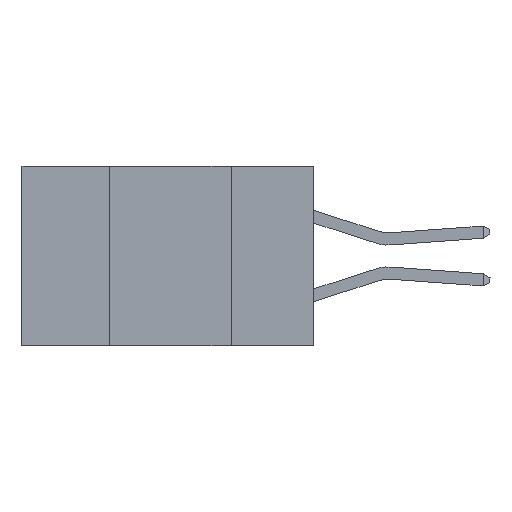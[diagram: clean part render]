
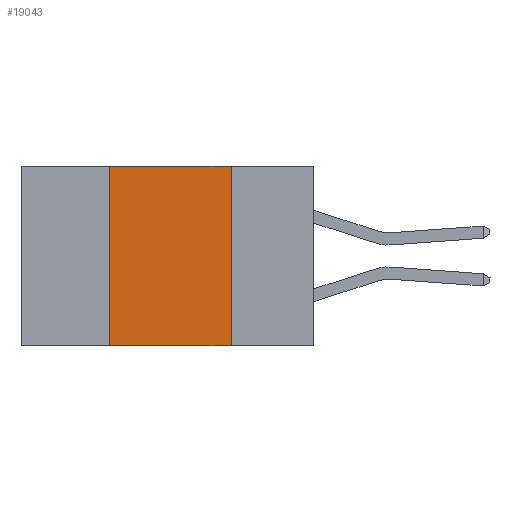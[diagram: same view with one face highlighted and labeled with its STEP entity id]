
A CAD part, left-side view. The second image highlights one B-rep face of the part: STEP entity #19043.
In plain terms, the highlighted planar face has unit normal (-1, 0, 0).
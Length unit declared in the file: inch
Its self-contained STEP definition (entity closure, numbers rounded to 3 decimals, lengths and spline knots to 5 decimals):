
#127 = VERTEX_POINT ( 'NONE', #21236 ) ;
#241 = ORIENTED_EDGE ( 'NONE', *, *, #1067, .F. ) ;
#625 = VECTOR ( 'NONE', #9538, 39.37008 ) ;
#987 = PLANE ( 'NONE',  #15501 ) ;
#1032 = LINE ( 'NONE', #20707, #12547 ) ;
#1067 = EDGE_CURVE ( 'NONE', #6345, #127, #12764, .T. ) ;
#2225 = CARTESIAN_POINT ( 'NONE',  ( 0., 0.17, 0. ) ) ;
#3621 = ORIENTED_EDGE ( 'NONE', *, *, #8249, .T. ) ;
#3716 = VECTOR ( 'NONE', #15698, 39.37008 ) ;
#3886 = EDGE_CURVE ( 'NONE', #127, #13129, #5242, .T. ) ;
#4466 = DIRECTION ( 'NONE',  ( 0., 0., -1. ) ) ;
#5242 = LINE ( 'NONE', #18087, #625 ) ;
#6345 = VERTEX_POINT ( 'NONE', #19664 ) ;
#7495 = DIRECTION ( 'NONE',  ( 0., 0., 1. ) ) ;
#8249 = EDGE_CURVE ( 'NONE', #6345, #10078, #17282, .T. ) ;
#8822 = DIRECTION ( 'NONE',  ( 0., 0., -1. ) ) ;
#9535 = ORIENTED_EDGE ( 'NONE', *, *, #3886, .F. ) ;
#9538 = DIRECTION ( 'NONE',  ( 0., -1., 0. ) ) ;
#10078 = VERTEX_POINT ( 'NONE', #14300 ) ;
#10540 = ORIENTED_EDGE ( 'NONE', *, *, #12432, .F. ) ;
#12310 = CARTESIAN_POINT ( 'NONE',  ( 0., 0.42, 0. ) ) ;
#12432 = EDGE_CURVE ( 'NONE', #13129, #10078, #1032, .T. ) ;
#12547 = VECTOR ( 'NONE', #8822, 39.37008 ) ;
#12764 = LINE ( 'NONE', #12310, #21149 ) ;
#12969 = CARTESIAN_POINT ( 'NONE',  ( 0., 0.6, 0. ) ) ;
#13129 = VERTEX_POINT ( 'NONE', #2225 ) ;
#13326 = FACE_OUTER_BOUND ( 'NONE', #15966, .T. ) ;
#14025 = CARTESIAN_POINT ( 'NONE',  ( 0., 0.6, -0.37 ) ) ;
#14300 = CARTESIAN_POINT ( 'NONE',  ( 0., 0.17, -0.37 ) ) ;
#14655 = DIRECTION ( 'NONE',  ( 1., 0., 0. ) ) ;
#15501 = AXIS2_PLACEMENT_3D ( 'NONE', #12969, #14655, #4466 ) ;
#15698 = DIRECTION ( 'NONE',  ( 0., -1., 0. ) ) ;
#15966 = EDGE_LOOP ( 'NONE', ( #10540, #9535, #241, #3621 ) ) ;
#17282 = LINE ( 'NONE', #14025, #3716 ) ;
#18087 = CARTESIAN_POINT ( 'NONE',  ( 0., 0.6, 0. ) ) ;
#19043 = ADVANCED_FACE ( 'NONE', ( #13326 ), #987, .F. ) ;
#19664 = CARTESIAN_POINT ( 'NONE',  ( 0., 0.42, -0.37 ) ) ;
#20707 = CARTESIAN_POINT ( 'NONE',  ( 0., 0.17, 0. ) ) ;
#21149 = VECTOR ( 'NONE', #7495, 39.37008 ) ;
#21236 = CARTESIAN_POINT ( 'NONE',  ( 0., 0.42, 0. ) ) ;
